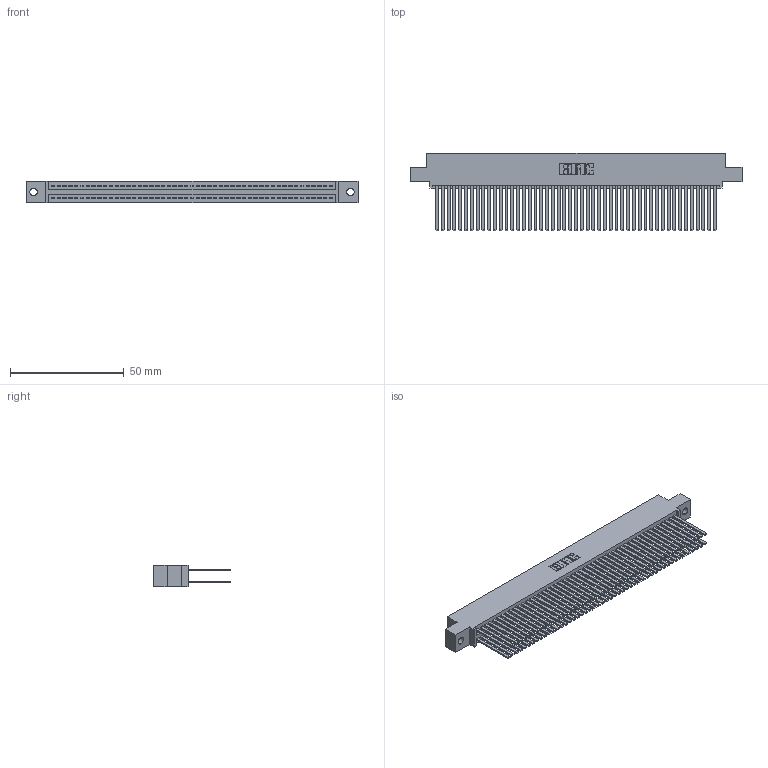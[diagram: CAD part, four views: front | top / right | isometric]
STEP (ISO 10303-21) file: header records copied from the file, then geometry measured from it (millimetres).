
FILE_DESCRIPTION (( 'STEP AP203' ), '1' );
FILE_NAME ('395-098-544-502.STEP', '2019-10-26T13:33:00', ( '' ), ( '' ), 'SwSTEP 2.0', 'SolidWorks 2016', '' );
FILE_SCHEMA (( 'CONFIG_CONTROL_DESIGN' ));
Length unit declared in the file: inch
Products named in the file (3): 345 Part_0.110 Offset - 0.128 Dia; 345-292-001_345-293-144; 395-098-544-502
Assembly tree (99 placements, depth 2):
  395-098-544-502
    345 Part_0.110 Offset - 0.128 Dia
    345-292-001_345-293-144  x98
Bounding box: 145.67 x 33.96 x 9.4 mm (x, y, z)
Volume: 15479.1 mm3; surface area: 26862.9 mm2
Topology: 99 solids, 99 shells, 4442 faces, 13191 edges, 8662 vertices
Faces by surface type: plane 2926, cylinder 1516
Entity records: 37455 total; most frequent: CARTESIAN_POINT 6272, ORIENTED_EDGE 6206, DIRECTION 5519, EDGE_CURVE 3103, VECTOR 2779, LINE 2779, VERTEX_POINT 2066, AXIS2_PLACEMENT_3D 1370
